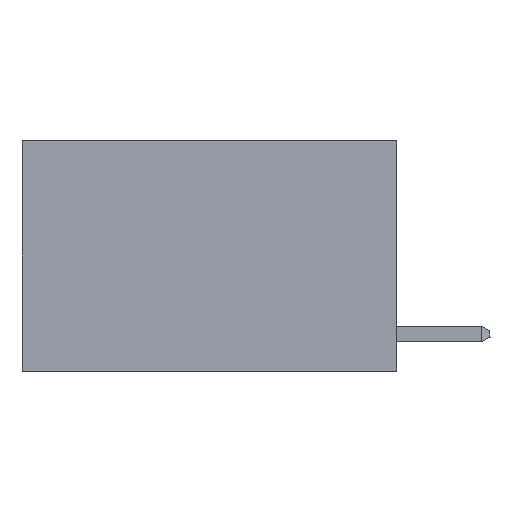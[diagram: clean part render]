
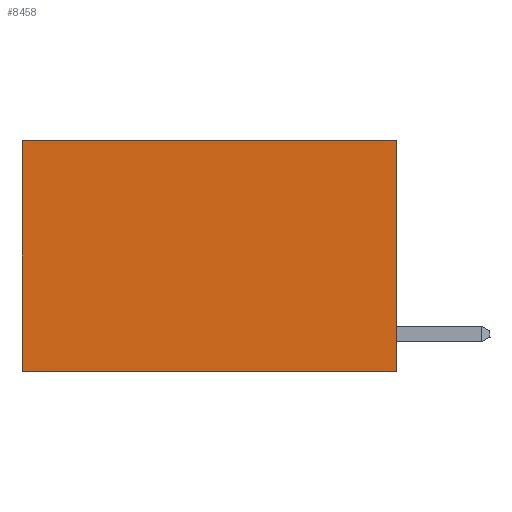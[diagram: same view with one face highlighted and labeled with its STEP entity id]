
A CAD part, left-side view. The second image highlights one B-rep face of the part: STEP entity #8458.
In plain terms, the highlighted planar face has unit normal (-1, 0, 0).
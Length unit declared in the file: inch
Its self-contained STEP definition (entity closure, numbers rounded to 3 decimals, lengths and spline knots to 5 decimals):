
#199 = FACE_OUTER_BOUND ( 'NONE', #4988, .T. ) ;
#904 = DIRECTION ( 'NONE',  ( 0., 1., 0. ) ) ;
#1023 = VERTEX_POINT ( 'NONE', #6804 ) ;
#1097 = CARTESIAN_POINT ( 'NONE',  ( 0.2625, 0., -0.37 ) ) ;
#1297 = DIRECTION ( 'NONE',  ( 0., 1., 0. ) ) ;
#1506 = VERTEX_POINT ( 'NONE', #3760 ) ;
#1827 = EDGE_CURVE ( 'NONE', #1506, #2831, #10360, .T. ) ;
#2261 = EDGE_CURVE ( 'NONE', #2831, #1023, #4863, .T. ) ;
#2831 = VERTEX_POINT ( 'NONE', #1097 ) ;
#2940 = LINE ( 'NONE', #7236, #6741 ) ;
#3203 = VECTOR ( 'NONE', #9826, 39.37008 ) ;
#3204 = LINE ( 'NONE', #6503, #3203 ) ;
#3224 = ORIENTED_EDGE ( 'NONE', *, *, #4664, .T. ) ;
#3436 = AXIS2_PLACEMENT_3D ( 'NONE', #3540, #4139, #7461 ) ;
#3540 = CARTESIAN_POINT ( 'NONE',  ( 0.2625, 0., 0. ) ) ;
#3760 = CARTESIAN_POINT ( 'NONE',  ( 0.2625, 0., 0. ) ) ;
#4139 = DIRECTION ( 'NONE',  ( 1., 0., 0. ) ) ;
#4664 = EDGE_CURVE ( 'NONE', #1506, #10417, #2940, .T. ) ;
#4744 = CARTESIAN_POINT ( 'NONE',  ( 0.2625, 0.6, 0. ) ) ;
#4863 = LINE ( 'NONE', #9807, #9841 ) ;
#4988 = EDGE_LOOP ( 'NONE', ( #6213, #5821, #7319, #3224 ) ) ;
#5408 = DIRECTION ( 'NONE',  ( 0., 0., -1. ) ) ;
#5821 = ORIENTED_EDGE ( 'NONE', *, *, #2261, .F. ) ;
#6040 = EDGE_CURVE ( 'NONE', #10417, #1023, #3204, .T. ) ;
#6213 = ORIENTED_EDGE ( 'NONE', *, *, #6040, .T. ) ;
#6475 = VECTOR ( 'NONE', #5408, 39.37008 ) ;
#6503 = CARTESIAN_POINT ( 'NONE',  ( 0.2625, 0.6, 0. ) ) ;
#6741 = VECTOR ( 'NONE', #1297, 39.37008 ) ;
#6804 = CARTESIAN_POINT ( 'NONE',  ( 0.2625, 0.6, -0.37 ) ) ;
#6992 = CARTESIAN_POINT ( 'NONE',  ( 0.2625, 0., 0. ) ) ;
#7236 = CARTESIAN_POINT ( 'NONE',  ( 0.2625, 0., 0. ) ) ;
#7319 = ORIENTED_EDGE ( 'NONE', *, *, #1827, .F. ) ;
#7461 = DIRECTION ( 'NONE',  ( 0., 0., -1. ) ) ;
#8267 = PLANE ( 'NONE',  #3436 ) ;
#8458 = ADVANCED_FACE ( 'NONE', ( #199 ), #8267, .F. ) ;
#9807 = CARTESIAN_POINT ( 'NONE',  ( 0.2625, 0., -0.37 ) ) ;
#9826 = DIRECTION ( 'NONE',  ( 0., 0., -1. ) ) ;
#9841 = VECTOR ( 'NONE', #904, 39.37008 ) ;
#10360 = LINE ( 'NONE', #6992, #6475 ) ;
#10417 = VERTEX_POINT ( 'NONE', #4744 ) ;
